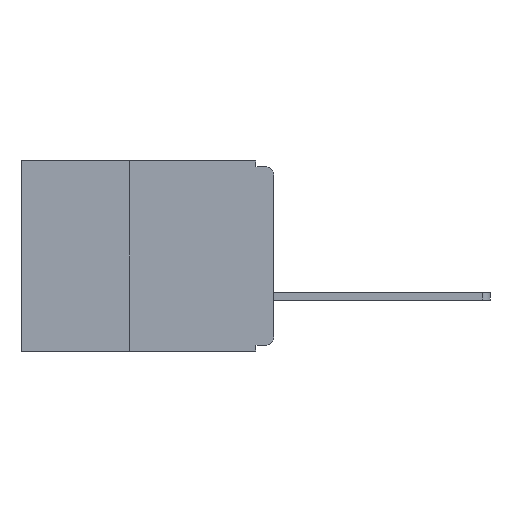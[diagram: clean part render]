
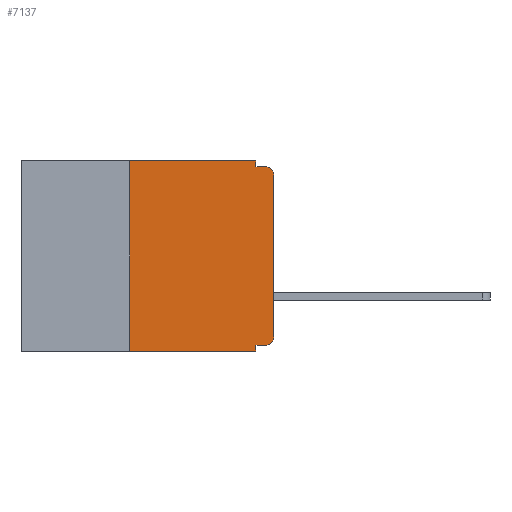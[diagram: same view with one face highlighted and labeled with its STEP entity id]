
A CAD part, left-side view. The second image highlights one B-rep face of the part: STEP entity #7137.
In plain terms, the highlighted planar face has unit normal (-1, 0, 0).
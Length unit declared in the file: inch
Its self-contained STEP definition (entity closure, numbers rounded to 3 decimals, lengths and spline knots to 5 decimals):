
#575 = VERTEX_POINT ( 'NONE', #11977 ) ;
#1066 = CARTESIAN_POINT ( 'NONE',  ( 0., 0.031, 0. ) ) ;
#1144 = LINE ( 'NONE', #12464, #19380 ) ;
#1720 = CIRCLE ( 'NONE', #11308, 0.015 ) ;
#2191 = EDGE_CURVE ( 'NONE', #6588, #18698, #17762, .T. ) ;
#2616 = ORIENTED_EDGE ( 'NONE', *, *, #22778, .F. ) ;
#2829 = LINE ( 'NONE', #14134, #6592 ) ;
#3192 = CARTESIAN_POINT ( 'NONE',  ( 0., 0.015, -0.32 ) ) ;
#3361 = ORIENTED_EDGE ( 'NONE', *, *, #4433, .F. ) ;
#3590 = AXIS2_PLACEMENT_3D ( 'NONE', #4566, #20930, #10182 ) ;
#3696 = CARTESIAN_POINT ( 'NONE',  ( 0., 0.015, -0.025 ) ) ;
#3777 = EDGE_CURVE ( 'NONE', #10355, #6804, #7517, .T. ) ;
#3924 = VECTOR ( 'NONE', #10022, 39.37008 ) ;
#4433 = EDGE_CURVE ( 'NONE', #575, #6588, #17390, .T. ) ;
#4566 = CARTESIAN_POINT ( 'NONE',  ( 0., 0.437, 0. ) ) ;
#5540 = DIRECTION ( 'NONE',  ( 0., 0., -1. ) ) ;
#5729 = ORIENTED_EDGE ( 'NONE', *, *, #17630, .F. ) ;
#5889 = VECTOR ( 'NONE', #12109, 39.37008 ) ;
#5920 = VECTOR ( 'NONE', #11560, 39.37008 ) ;
#6588 = VERTEX_POINT ( 'NONE', #9348 ) ;
#6592 = VECTOR ( 'NONE', #15960, 39.37008 ) ;
#6804 = VERTEX_POINT ( 'NONE', #17137 ) ;
#6870 = CIRCLE ( 'NONE', #9077, 0.015 ) ;
#6914 = ORIENTED_EDGE ( 'NONE', *, *, #15876, .F. ) ;
#6987 = VERTEX_POINT ( 'NONE', #13340 ) ;
#7126 = DIRECTION ( 'NONE',  ( 0., 0., 1. ) ) ;
#7137 = ADVANCED_FACE ( 'NONE', ( #16432 ), #8366, .F. ) ;
#7282 = CARTESIAN_POINT ( 'NONE',  ( 0., 0., 0. ) ) ;
#7517 = LINE ( 'NONE', #7282, #16566 ) ;
#7776 = DIRECTION ( 'NONE',  ( -1., 0., 0. ) ) ;
#8185 = CARTESIAN_POINT ( 'NONE',  ( 0., 0.437, 0. ) ) ;
#8323 = VERTEX_POINT ( 'NONE', #16994 ) ;
#8366 = PLANE ( 'NONE',  #3590 ) ;
#9077 = AXIS2_PLACEMENT_3D ( 'NONE', #18584, #7776, #20362 ) ;
#9348 = CARTESIAN_POINT ( 'NONE',  ( 0., 0.031, -0.01 ) ) ;
#9926 = VERTEX_POINT ( 'NONE', #3192 ) ;
#10022 = DIRECTION ( 'NONE',  ( 0., -1., 0. ) ) ;
#10182 = DIRECTION ( 'NONE',  ( 0., 0., -1. ) ) ;
#10291 = LINE ( 'NONE', #22277, #5920 ) ;
#10355 = VERTEX_POINT ( 'NONE', #19094 ) ;
#10878 = ORIENTED_EDGE ( 'NONE', *, *, #22085, .T. ) ;
#11308 = AXIS2_PLACEMENT_3D ( 'NONE', #3696, #16477, #5540 ) ;
#11416 = ORIENTED_EDGE ( 'NONE', *, *, #2191, .F. ) ;
#11560 = DIRECTION ( 'NONE',  ( 0., 1., 0. ) ) ;
#11977 = CARTESIAN_POINT ( 'NONE',  ( 0., 0.031, 0. ) ) ;
#12109 = DIRECTION ( 'NONE',  ( 0., 0., 1. ) ) ;
#12126 = DIRECTION ( 'NONE',  ( 0., 0., -1. ) ) ;
#12464 = CARTESIAN_POINT ( 'NONE',  ( 0., 0.437, -0.33 ) ) ;
#12538 = DIRECTION ( 'NONE',  ( 0., -1., 0. ) ) ;
#13340 = CARTESIAN_POINT ( 'NONE',  ( 0., 0.25, -0.33 ) ) ;
#13732 = EDGE_CURVE ( 'NONE', #6987, #8323, #1144, .T. ) ;
#14134 = CARTESIAN_POINT ( 'NONE',  ( 0., 0.031, -0.33 ) ) ;
#14791 = CARTESIAN_POINT ( 'NONE',  ( 0., 0., -0.01 ) ) ;
#15060 = EDGE_CURVE ( 'NONE', #6804, #18698, #1720, .T. ) ;
#15076 = ORIENTED_EDGE ( 'NONE', *, *, #22235, .F. ) ;
#15876 = EDGE_CURVE ( 'NONE', #16372, #8323, #2829, .T. ) ;
#15960 = DIRECTION ( 'NONE',  ( 0., 0., -1. ) ) ;
#16000 = VERTEX_POINT ( 'NONE', #19907 ) ;
#16372 = VERTEX_POINT ( 'NONE', #21005 ) ;
#16432 = FACE_OUTER_BOUND ( 'NONE', #21304, .T. ) ;
#16477 = DIRECTION ( 'NONE',  ( -1., 0., 0. ) ) ;
#16566 = VECTOR ( 'NONE', #7126, 39.37008 ) ;
#16994 = CARTESIAN_POINT ( 'NONE',  ( 0., 0.031, -0.33 ) ) ;
#17137 = CARTESIAN_POINT ( 'NONE',  ( 0., 0., -0.025 ) ) ;
#17390 = LINE ( 'NONE', #1066, #21575 ) ;
#17630 = EDGE_CURVE ( 'NONE', #6987, #16000, #20357, .T. ) ;
#17762 = LINE ( 'NONE', #14791, #22489 ) ;
#18380 = ORIENTED_EDGE ( 'NONE', *, *, #13732, .T. ) ;
#18584 = CARTESIAN_POINT ( 'NONE',  ( 0., 0.015, -0.305 ) ) ;
#18698 = VERTEX_POINT ( 'NONE', #20992 ) ;
#18780 = ORIENTED_EDGE ( 'NONE', *, *, #15060, .T. ) ;
#19094 = CARTESIAN_POINT ( 'NONE',  ( 0., 0., -0.305 ) ) ;
#19380 = VECTOR ( 'NONE', #21382, 39.37008 ) ;
#19907 = CARTESIAN_POINT ( 'NONE',  ( 0., 0.25, 0. ) ) ;
#20357 = LINE ( 'NONE', #20869, #5889 ) ;
#20362 = DIRECTION ( 'NONE',  ( 0., 0., -1. ) ) ;
#20869 = CARTESIAN_POINT ( 'NONE',  ( 0., 0.25, -0.33 ) ) ;
#20930 = DIRECTION ( 'NONE',  ( 1., 0., 0. ) ) ;
#20992 = CARTESIAN_POINT ( 'NONE',  ( 0., 0.015, -0.01 ) ) ;
#21005 = CARTESIAN_POINT ( 'NONE',  ( 0., 0.031, -0.32 ) ) ;
#21304 = EDGE_LOOP ( 'NONE', ( #21981, #18780, #11416, #3361, #15076, #5729, #18380, #6914, #2616, #10878 ) ) ;
#21382 = DIRECTION ( 'NONE',  ( 0., -1., 0. ) ) ;
#21575 = VECTOR ( 'NONE', #12126, 39.37008 ) ;
#21981 = ORIENTED_EDGE ( 'NONE', *, *, #3777, .T. ) ;
#22085 = EDGE_CURVE ( 'NONE', #9926, #10355, #6870, .T. ) ;
#22235 = EDGE_CURVE ( 'NONE', #16000, #575, #22635, .T. ) ;
#22277 = CARTESIAN_POINT ( 'NONE',  ( 0., 0., -0.32 ) ) ;
#22489 = VECTOR ( 'NONE', #12538, 39.37008 ) ;
#22635 = LINE ( 'NONE', #8185, #3924 ) ;
#22778 = EDGE_CURVE ( 'NONE', #9926, #16372, #10291, .T. ) ;
